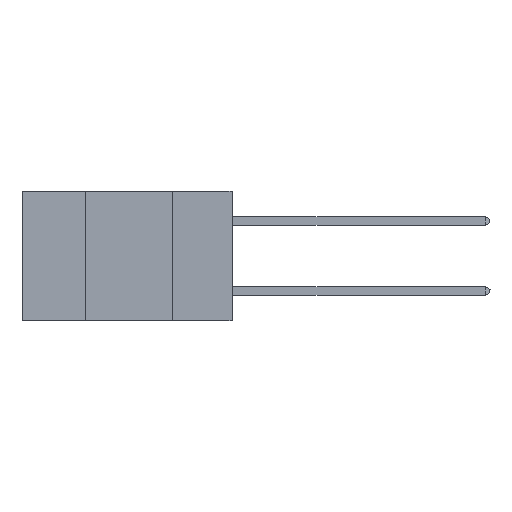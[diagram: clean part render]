
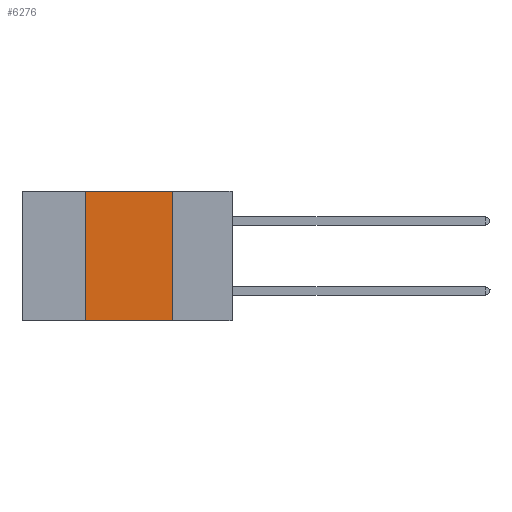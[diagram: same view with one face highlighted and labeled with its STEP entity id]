
A CAD part, left-side view. The second image highlights one B-rep face of the part: STEP entity #6276.
In plain terms, the highlighted planar face has unit normal (-1, 0, 0).
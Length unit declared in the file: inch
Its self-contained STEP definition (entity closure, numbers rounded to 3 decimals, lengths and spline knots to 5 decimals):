
#36 = VECTOR ( 'NONE', #322, 39.37008 ) ;
#60 = CARTESIAN_POINT ( 'NONE',  ( 0., 0.42, 0. ) ) ;
#322 = DIRECTION ( 'NONE',  ( 0., 0., 1. ) ) ;
#1386 = CARTESIAN_POINT ( 'NONE',  ( 0., 0.42, -0.37 ) ) ;
#1425 = LINE ( 'NONE', #3294, #22858 ) ;
#2295 = DIRECTION ( 'NONE',  ( 0., 0., -1. ) ) ;
#2629 = VERTEX_POINT ( 'NONE', #1386 ) ;
#3294 = CARTESIAN_POINT ( 'NONE',  ( 0., 0.6, 0. ) ) ;
#4868 = CARTESIAN_POINT ( 'NONE',  ( 0., 0.17, 0. ) ) ;
#5464 = LINE ( 'NONE', #20280, #36 ) ;
#6276 = ADVANCED_FACE ( 'NONE', ( #15899 ), #9736, .F. ) ;
#6483 = DIRECTION ( 'NONE',  ( 0., 0., -1. ) ) ;
#8006 = VECTOR ( 'NONE', #9831, 39.37008 ) ;
#9736 = PLANE ( 'NONE',  #19500 ) ;
#9831 = DIRECTION ( 'NONE',  ( 0., -1., 0. ) ) ;
#9832 = EDGE_CURVE ( 'NONE', #22242, #19574, #1425, .T. ) ;
#9910 = EDGE_LOOP ( 'NONE', ( #18731, #15166, #18724, #20022 ) ) ;
#14477 = EDGE_CURVE ( 'NONE', #2629, #22242, #5464, .T. ) ;
#15092 = EDGE_CURVE ( 'NONE', #2629, #15389, #19849, .T. ) ;
#15166 = ORIENTED_EDGE ( 'NONE', *, *, #9832, .F. ) ;
#15389 = VERTEX_POINT ( 'NONE', #19863 ) ;
#15820 = EDGE_CURVE ( 'NONE', #19574, #15389, #15912, .T. ) ;
#15899 = FACE_OUTER_BOUND ( 'NONE', #9910, .T. ) ;
#15912 = LINE ( 'NONE', #20094, #19009 ) ;
#18169 = DIRECTION ( 'NONE',  ( 0., -1., 0. ) ) ;
#18724 = ORIENTED_EDGE ( 'NONE', *, *, #14477, .F. ) ;
#18731 = ORIENTED_EDGE ( 'NONE', *, *, #15820, .F. ) ;
#19009 = VECTOR ( 'NONE', #2295, 39.37008 ) ;
#19500 = AXIS2_PLACEMENT_3D ( 'NONE', #20777, #21240, #6483 ) ;
#19574 = VERTEX_POINT ( 'NONE', #4868 ) ;
#19849 = LINE ( 'NONE', #22511, #8006 ) ;
#19863 = CARTESIAN_POINT ( 'NONE',  ( 0., 0.17, -0.37 ) ) ;
#20022 = ORIENTED_EDGE ( 'NONE', *, *, #15092, .T. ) ;
#20094 = CARTESIAN_POINT ( 'NONE',  ( 0., 0.17, 0. ) ) ;
#20280 = CARTESIAN_POINT ( 'NONE',  ( 0., 0.42, 0. ) ) ;
#20777 = CARTESIAN_POINT ( 'NONE',  ( 0., 0.6, 0. ) ) ;
#21240 = DIRECTION ( 'NONE',  ( 1., 0., 0. ) ) ;
#22242 = VERTEX_POINT ( 'NONE', #60 ) ;
#22511 = CARTESIAN_POINT ( 'NONE',  ( 0., 0.6, -0.37 ) ) ;
#22858 = VECTOR ( 'NONE', #18169, 39.37008 ) ;
